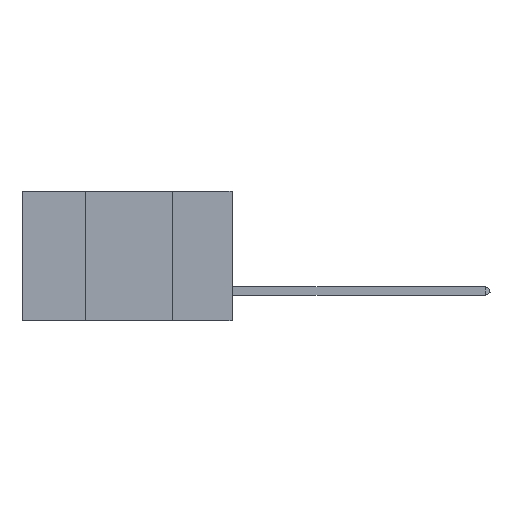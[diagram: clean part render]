
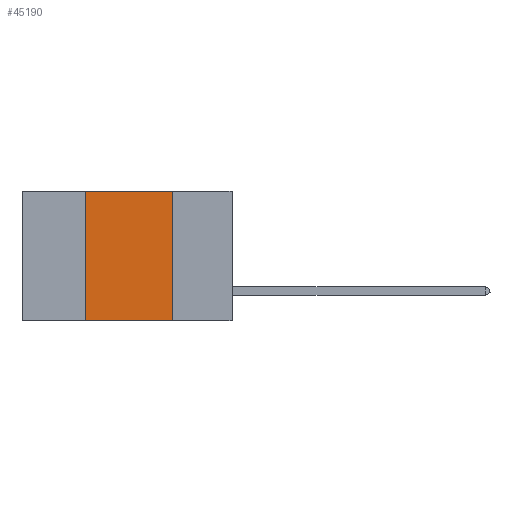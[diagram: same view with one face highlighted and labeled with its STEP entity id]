
A CAD part, left-side view. The second image highlights one B-rep face of the part: STEP entity #45190.
In plain terms, the highlighted planar face has unit normal (-1, 0, 0).
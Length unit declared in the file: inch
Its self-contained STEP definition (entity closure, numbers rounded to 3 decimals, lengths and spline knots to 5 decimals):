
#4284 = ORIENTED_EDGE ( 'NONE', *, *, #26165, .F. ) ;
#4404 = VECTOR ( 'NONE', #37552, 39.37008 ) ;
#4535 = VERTEX_POINT ( 'NONE', #9389 ) ;
#4810 = ORIENTED_EDGE ( 'NONE', *, *, #11180, .F. ) ;
#7911 = CARTESIAN_POINT ( 'NONE',  ( 0., 0.6, 0. ) ) ;
#8460 = VERTEX_POINT ( 'NONE', #46865 ) ;
#8843 = EDGE_LOOP ( 'NONE', ( #4284, #43560, #4810, #45965 ) ) ;
#9389 = CARTESIAN_POINT ( 'NONE',  ( 0., 0.17, -0.37 ) ) ;
#10605 = EDGE_CURVE ( 'NONE', #47113, #42196, #29884, .T. ) ;
#11180 = EDGE_CURVE ( 'NONE', #8460, #47113, #28674, .T. ) ;
#12519 = LINE ( 'NONE', #27148, #4404 ) ;
#12724 = DIRECTION ( 'NONE',  ( 0., 0., 1. ) ) ;
#13263 = VECTOR ( 'NONE', #29356, 39.37008 ) ;
#13534 = CARTESIAN_POINT ( 'NONE',  ( 0., 0.17, 0. ) ) ;
#13899 = EDGE_CURVE ( 'NONE', #8460, #4535, #17926, .T. ) ;
#14699 = VECTOR ( 'NONE', #12724, 39.37008 ) ;
#16657 = CARTESIAN_POINT ( 'NONE',  ( 0., 0.6, 0. ) ) ;
#16979 = DIRECTION ( 'NONE',  ( 1., 0., 0. ) ) ;
#17926 = LINE ( 'NONE', #33071, #13263 ) ;
#26165 = EDGE_CURVE ( 'NONE', #42196, #4535, #12519, .T. ) ;
#27148 = CARTESIAN_POINT ( 'NONE',  ( 0., 0.17, 0. ) ) ;
#28674 = LINE ( 'NONE', #30742, #14699 ) ;
#29356 = DIRECTION ( 'NONE',  ( 0., -1., 0. ) ) ;
#29884 = LINE ( 'NONE', #7911, #31051 ) ;
#30742 = CARTESIAN_POINT ( 'NONE',  ( 0., 0.42, 0. ) ) ;
#31051 = VECTOR ( 'NONE', #33895, 39.37008 ) ;
#31728 = PLANE ( 'NONE',  #41575 ) ;
#31865 = CARTESIAN_POINT ( 'NONE',  ( 0., 0.42, 0. ) ) ;
#33071 = CARTESIAN_POINT ( 'NONE',  ( 0., 0.6, -0.37 ) ) ;
#33895 = DIRECTION ( 'NONE',  ( 0., -1., 0. ) ) ;
#37552 = DIRECTION ( 'NONE',  ( 0., 0., -1. ) ) ;
#39478 = DIRECTION ( 'NONE',  ( 0., 0., -1. ) ) ;
#41575 = AXIS2_PLACEMENT_3D ( 'NONE', #16657, #16979, #39478 ) ;
#42196 = VERTEX_POINT ( 'NONE', #13534 ) ;
#43560 = ORIENTED_EDGE ( 'NONE', *, *, #10605, .F. ) ;
#45190 = ADVANCED_FACE ( 'NONE', ( #47599 ), #31728, .F. ) ;
#45965 = ORIENTED_EDGE ( 'NONE', *, *, #13899, .T. ) ;
#46865 = CARTESIAN_POINT ( 'NONE',  ( 0., 0.42, -0.37 ) ) ;
#47113 = VERTEX_POINT ( 'NONE', #31865 ) ;
#47599 = FACE_OUTER_BOUND ( 'NONE', #8843, .T. ) ;
